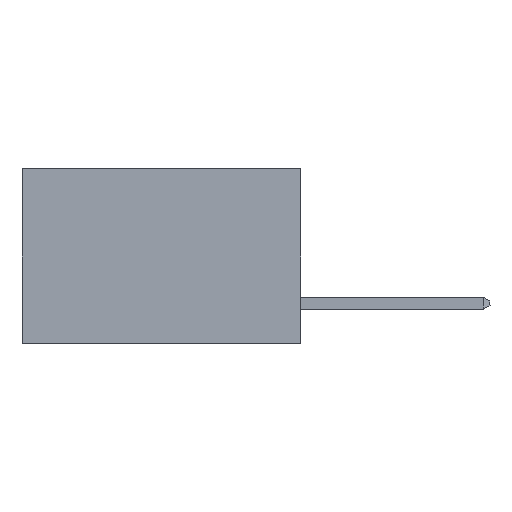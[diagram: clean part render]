
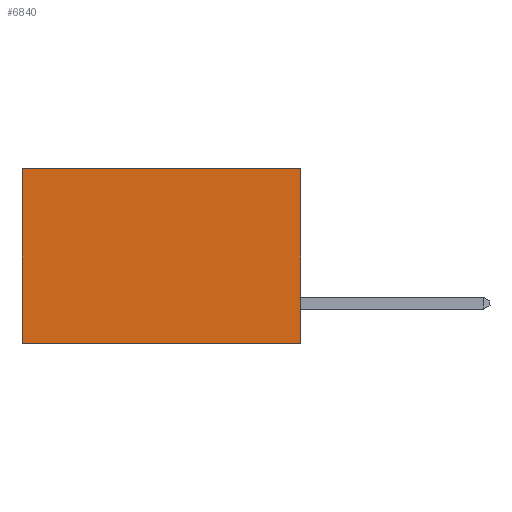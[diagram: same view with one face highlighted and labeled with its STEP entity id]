
A CAD part, left-side view. The second image highlights one B-rep face of the part: STEP entity #6840.
In plain terms, the highlighted planar face has unit normal (-1, 0, 0).
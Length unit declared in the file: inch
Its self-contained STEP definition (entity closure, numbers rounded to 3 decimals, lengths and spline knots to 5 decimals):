
#89 = LINE ( 'NONE', #4820, #4867 ) ;
#146 = AXIS2_PLACEMENT_3D ( 'NONE', #9207, #9182, #9016 ) ;
#1690 = CARTESIAN_POINT ( 'NONE',  ( 0.277, 0., -0.37 ) ) ;
#1839 = EDGE_CURVE ( 'NONE', #2193, #11680, #2740, .T. ) ;
#2013 = CARTESIAN_POINT ( 'NONE',  ( 0.277, 0.59, -0.37 ) ) ;
#2193 = VERTEX_POINT ( 'NONE', #10345 ) ;
#2277 = CARTESIAN_POINT ( 'NONE',  ( 0.277, 0., 0. ) ) ;
#2558 = ORIENTED_EDGE ( 'NONE', *, *, #1839, .F. ) ;
#2740 = LINE ( 'NONE', #9830, #7360 ) ;
#2994 = VECTOR ( 'NONE', #10053, 39.37008 ) ;
#3551 = DIRECTION ( 'NONE',  ( 0., 0., -1. ) ) ;
#4770 = DIRECTION ( 'NONE',  ( 0., 0., -1. ) ) ;
#4820 = CARTESIAN_POINT ( 'NONE',  ( 0.277, 0.59, -0.37 ) ) ;
#4867 = VECTOR ( 'NONE', #4770, 39.37008 ) ;
#6840 = ADVANCED_FACE ( 'NONE', ( #7973 ), #9393, .F. ) ;
#6877 = DIRECTION ( 'NONE',  ( 0., 1., 0. ) ) ;
#6884 = ORIENTED_EDGE ( 'NONE', *, *, #7083, .T. ) ;
#7083 = EDGE_CURVE ( 'NONE', #10561, #7843, #89, .T. ) ;
#7360 = VECTOR ( 'NONE', #3551, 39.37008 ) ;
#7465 = ORIENTED_EDGE ( 'NONE', *, *, #11023, .T. ) ;
#7843 = VERTEX_POINT ( 'NONE', #2013 ) ;
#7854 = VECTOR ( 'NONE', #6877, 39.37008 ) ;
#7855 = CARTESIAN_POINT ( 'NONE',  ( 0.277, 0.59, 0. ) ) ;
#7973 = FACE_OUTER_BOUND ( 'NONE', #11276, .T. ) ;
#8147 = LINE ( 'NONE', #2277, #7854 ) ;
#9016 = DIRECTION ( 'NONE',  ( 0., 0., -1. ) ) ;
#9182 = DIRECTION ( 'NONE',  ( 1., 0., 0. ) ) ;
#9207 = CARTESIAN_POINT ( 'NONE',  ( 0.277, 0., -0.37 ) ) ;
#9393 = PLANE ( 'NONE',  #146 ) ;
#9830 = CARTESIAN_POINT ( 'NONE',  ( 0.277, 0., -0.37 ) ) ;
#10053 = DIRECTION ( 'NONE',  ( 0., 1., 0. ) ) ;
#10214 = EDGE_CURVE ( 'NONE', #11680, #7843, #10470, .T. ) ;
#10345 = CARTESIAN_POINT ( 'NONE',  ( 0.277, 0., 0. ) ) ;
#10470 = LINE ( 'NONE', #1690, #2994 ) ;
#10561 = VERTEX_POINT ( 'NONE', #7855 ) ;
#11023 = EDGE_CURVE ( 'NONE', #2193, #10561, #8147, .T. ) ;
#11276 = EDGE_LOOP ( 'NONE', ( #6884, #11564, #2558, #7465 ) ) ;
#11315 = CARTESIAN_POINT ( 'NONE',  ( 0.277, 0., -0.37 ) ) ;
#11564 = ORIENTED_EDGE ( 'NONE', *, *, #10214, .F. ) ;
#11680 = VERTEX_POINT ( 'NONE', #11315 ) ;
